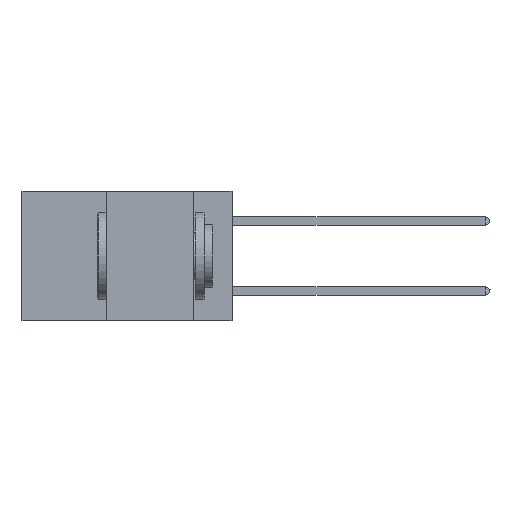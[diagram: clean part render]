
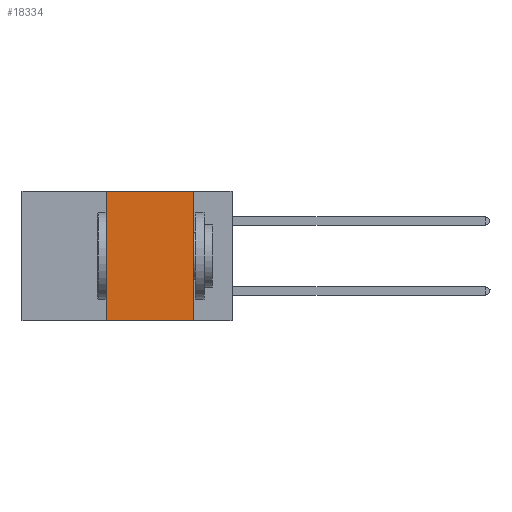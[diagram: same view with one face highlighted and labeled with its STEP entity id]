
A CAD part, left-side view. The second image highlights one B-rep face of the part: STEP entity #18334.
In plain terms, the highlighted planar face has unit normal (-1, 0, 0).
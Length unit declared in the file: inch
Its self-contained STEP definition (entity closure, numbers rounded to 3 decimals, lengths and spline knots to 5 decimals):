
#2180 = DIRECTION ( 'NONE',  ( 0., -1., 0. ) ) ;
#2795 = VERTEX_POINT ( 'NONE', #8544 ) ;
#4596 = VECTOR ( 'NONE', #12314, 39.37008 ) ;
#6680 = LINE ( 'NONE', #9352, #12942 ) ;
#6990 = CARTESIAN_POINT ( 'NONE',  ( 0., 0.36, 0. ) ) ;
#8544 = CARTESIAN_POINT ( 'NONE',  ( 0., 0.11, -0.37 ) ) ;
#8663 = VERTEX_POINT ( 'NONE', #10655 ) ;
#9210 = VECTOR ( 'NONE', #9730, 39.37008 ) ;
#9352 = CARTESIAN_POINT ( 'NONE',  ( 0., 0.36, 0. ) ) ;
#9730 = DIRECTION ( 'NONE',  ( 0., 0., -1. ) ) ;
#10512 = AXIS2_PLACEMENT_3D ( 'NONE', #12739, #37330, #28302 ) ;
#10655 = CARTESIAN_POINT ( 'NONE',  ( 0., 0.36, -0.37 ) ) ;
#12314 = DIRECTION ( 'NONE',  ( 0., -1., 0. ) ) ;
#12739 = CARTESIAN_POINT ( 'NONE',  ( 0., 0.6, 0. ) ) ;
#12942 = VECTOR ( 'NONE', #27855, 39.37008 ) ;
#14099 = EDGE_CURVE ( 'NONE', #8663, #25732, #6680, .T. ) ;
#14574 = CARTESIAN_POINT ( 'NONE',  ( 0., 0.11, 0. ) ) ;
#15259 = VERTEX_POINT ( 'NONE', #14574 ) ;
#15608 = ORIENTED_EDGE ( 'NONE', *, *, #17740, .F. ) ;
#17740 = EDGE_CURVE ( 'NONE', #25732, #15259, #20976, .T. ) ;
#18272 = EDGE_LOOP ( 'NONE', ( #34695, #15608, #31873, #39254 ) ) ;
#18334 = ADVANCED_FACE ( 'NONE', ( #33384 ), #22034, .F. ) ;
#20976 = LINE ( 'NONE', #30681, #4596 ) ;
#22034 = PLANE ( 'NONE',  #10512 ) ;
#24869 = CARTESIAN_POINT ( 'NONE',  ( 0., 0.11, 0. ) ) ;
#25404 = EDGE_CURVE ( 'NONE', #8663, #2795, #38004, .T. ) ;
#25732 = VERTEX_POINT ( 'NONE', #6990 ) ;
#27855 = DIRECTION ( 'NONE',  ( 0., 0., 1. ) ) ;
#28302 = DIRECTION ( 'NONE',  ( 0., 0., -1. ) ) ;
#30681 = CARTESIAN_POINT ( 'NONE',  ( 0., 0.6, 0. ) ) ;
#31873 = ORIENTED_EDGE ( 'NONE', *, *, #14099, .F. ) ;
#33336 = EDGE_CURVE ( 'NONE', #15259, #2795, #33670, .T. ) ;
#33384 = FACE_OUTER_BOUND ( 'NONE', #18272, .T. ) ;
#33670 = LINE ( 'NONE', #24869, #9210 ) ;
#34695 = ORIENTED_EDGE ( 'NONE', *, *, #33336, .F. ) ;
#35144 = VECTOR ( 'NONE', #2180, 39.37008 ) ;
#37330 = DIRECTION ( 'NONE',  ( 1., 0., 0. ) ) ;
#38004 = LINE ( 'NONE', #38624, #35144 ) ;
#38624 = CARTESIAN_POINT ( 'NONE',  ( 0., 0.6, -0.37 ) ) ;
#39254 = ORIENTED_EDGE ( 'NONE', *, *, #25404, .T. ) ;
